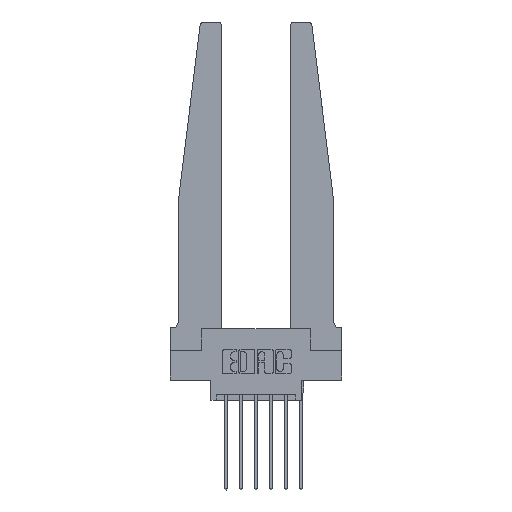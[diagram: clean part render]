
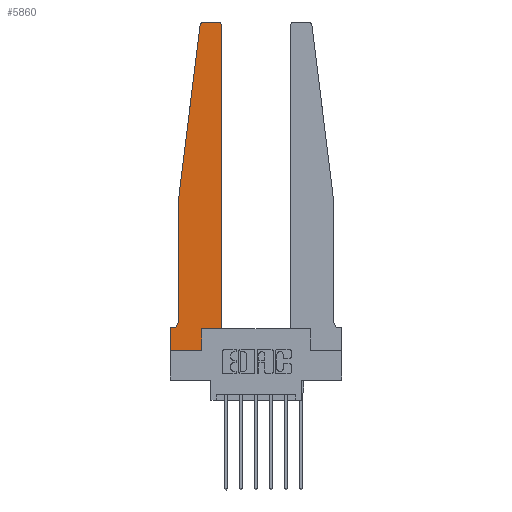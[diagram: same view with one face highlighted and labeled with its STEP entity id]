
A CAD part, top view. The second image highlights one B-rep face of the part: STEP entity #5860.
In plain terms, the highlighted planar face has unit normal (0, 0, 1).
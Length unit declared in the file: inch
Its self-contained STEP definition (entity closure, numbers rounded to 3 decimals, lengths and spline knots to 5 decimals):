
#314 = CIRCLE ( 'NONE', #8016, 0.03 ) ;
#333 = CARTESIAN_POINT ( 'NONE',  ( 0.24675, 2.72367, 0.37 ) ) ;
#404 = VERTEX_POINT ( 'NONE', #2735 ) ;
#415 = ORIENTED_EDGE ( 'NONE', *, *, #5354, .T. ) ;
#635 = DIRECTION ( 'NONE',  ( 0., 0., 1. ) ) ;
#674 = EDGE_CURVE ( 'NONE', #12169, #11411, #849, .T. ) ;
#849 = CIRCLE ( 'NONE', #8551, 0.03 ) ;
#889 = CARTESIAN_POINT ( 'NONE',  ( 0., 0.1875, 0.37 ) ) ;
#920 = VECTOR ( 'NONE', #7276, 39.37008 ) ;
#926 = CARTESIAN_POINT ( 'NONE',  ( 0.015, 0.2375, 0.37 ) ) ;
#1264 = EDGE_CURVE ( 'NONE', #7912, #12169, #11225, .T. ) ;
#1346 = ORIENTED_EDGE ( 'NONE', *, *, #674, .T. ) ;
#1358 = AXIS2_PLACEMENT_3D ( 'NONE', #926, #13428, #7123 ) ;
#1378 = CARTESIAN_POINT ( 'NONE',  ( 0.2605, 0.18, 0.37 ) ) ;
#1619 = LINE ( 'NONE', #10051, #3954 ) ;
#1695 = DIRECTION ( 'NONE',  ( -0.122, -0.992, 0. ) ) ;
#1724 = LINE ( 'NONE', #10158, #8013 ) ;
#1923 = DIRECTION ( 'NONE',  ( 0., 0., 1. ) ) ;
#2057 = FACE_OUTER_BOUND ( 'NONE', #11033, .T. ) ;
#2199 = VERTEX_POINT ( 'NONE', #4110 ) ;
#2253 = DIRECTION ( 'NONE',  ( 1., 0., 0. ) ) ;
#2413 = DIRECTION ( 'NONE',  ( 0., 1., 0. ) ) ;
#2567 = DIRECTION ( 'NONE',  ( 0., -1., 0. ) ) ;
#2568 = CARTESIAN_POINT ( 'NONE',  ( 0.2605, 0., 0.37 ) ) ;
#2637 = LINE ( 'NONE', #3870, #7713 ) ;
#2700 = ORIENTED_EDGE ( 'NONE', *, *, #9136, .T. ) ;
#2715 = LINE ( 'NONE', #3741, #9560 ) ;
#2735 = CARTESIAN_POINT ( 'NONE',  ( 0., 0., 0.37 ) ) ;
#2786 = ORIENTED_EDGE ( 'NONE', *, *, #4569, .T. ) ;
#2891 = CARTESIAN_POINT ( 'NONE',  ( 0.2605, 0.18, 0.37 ) ) ;
#3127 = CARTESIAN_POINT ( 'NONE',  ( 0.27653, 2.75, 0.37 ) ) ;
#3148 = PLANE ( 'NONE',  #8619 ) ;
#3382 = ORIENTED_EDGE ( 'NONE', *, *, #9027, .T. ) ;
#3513 = VECTOR ( 'NONE', #13382, 39.37008 ) ;
#3741 = CARTESIAN_POINT ( 'NONE',  ( 0.425, 0.18, 0.37 ) ) ;
#3796 = CARTESIAN_POINT ( 'NONE',  ( 0.27653, 2.72, 0.37 ) ) ;
#3854 = ORIENTED_EDGE ( 'NONE', *, *, #1264, .T. ) ;
#3870 = CARTESIAN_POINT ( 'NONE',  ( 0.065, 1.25, 0.37 ) ) ;
#3954 = VECTOR ( 'NONE', #2567, 39.37008 ) ;
#4041 = CARTESIAN_POINT ( 'NONE',  ( 0., 0.1875, 0.37 ) ) ;
#4102 = DIRECTION ( 'NONE',  ( 0., 0., 1. ) ) ;
#4110 = CARTESIAN_POINT ( 'NONE',  ( 0.425, 0.18, 0.37 ) ) ;
#4569 = EDGE_CURVE ( 'NONE', #5916, #404, #1619, .T. ) ;
#4619 = EDGE_CURVE ( 'NONE', #11189, #12690, #2637, .T. ) ;
#4818 = LINE ( 'NONE', #11382, #6033 ) ;
#4831 = DIRECTION ( 'NONE',  ( 1., 0., 0. ) ) ;
#5354 = EDGE_CURVE ( 'NONE', #12690, #12303, #10393, .T. ) ;
#5358 = CARTESIAN_POINT ( 'NONE',  ( 0.395, 2.72, 0.37 ) ) ;
#5711 = EDGE_CURVE ( 'NONE', #12443, #11377, #12017, .T. ) ;
#5774 = ORIENTED_EDGE ( 'NONE', *, *, #12333, .T. ) ;
#5860 = ADVANCED_FACE ( 'NONE', ( #2057 ), #3148, .T. ) ;
#5876 = DIRECTION ( 'NONE',  ( 0., -1., 0. ) ) ;
#5877 = DIRECTION ( 'NONE',  ( 0., 1., 0. ) ) ;
#5916 = VERTEX_POINT ( 'NONE', #4041 ) ;
#5963 = CARTESIAN_POINT ( 'NONE',  ( 0.065, 1.25, 0.37 ) ) ;
#6033 = VECTOR ( 'NONE', #13664, 39.37008 ) ;
#6263 = EDGE_CURVE ( 'NONE', #11377, #2199, #12470, .T. ) ;
#6335 = VERTEX_POINT ( 'NONE', #9221 ) ;
#7123 = DIRECTION ( 'NONE',  ( -1., 0., 0. ) ) ;
#7276 = DIRECTION ( 'NONE',  ( 1., 0., 0. ) ) ;
#7650 = EDGE_CURVE ( 'NONE', #11411, #11189, #9139, .T. ) ;
#7713 = VECTOR ( 'NONE', #5876, 39.37008 ) ;
#7912 = VERTEX_POINT ( 'NONE', #9551 ) ;
#7988 = DIRECTION ( 'NONE',  ( -1., 0., 0. ) ) ;
#8013 = VECTOR ( 'NONE', #7988, 39.37008 ) ;
#8016 = AXIS2_PLACEMENT_3D ( 'NONE', #5358, #4102, #2253 ) ;
#8194 = DIRECTION ( 'NONE',  ( 1., 0., 0. ) ) ;
#8215 = CARTESIAN_POINT ( 'NONE',  ( 0.065, 1.25, 0.37 ) ) ;
#8289 = ORIENTED_EDGE ( 'NONE', *, *, #4619, .T. ) ;
#8392 = ORIENTED_EDGE ( 'NONE', *, *, #12643, .T. ) ;
#8551 = AXIS2_PLACEMENT_3D ( 'NONE', #3796, #635, #4831 ) ;
#8619 = AXIS2_PLACEMENT_3D ( 'NONE', #889, #1923, #8194 ) ;
#9027 = EDGE_CURVE ( 'NONE', #12303, #5916, #1724, .T. ) ;
#9136 = EDGE_CURVE ( 'NONE', #404, #12443, #4818, .T. ) ;
#9139 = LINE ( 'NONE', #5963, #13528 ) ;
#9221 = CARTESIAN_POINT ( 'NONE',  ( 0.425, 2.72, 0.37 ) ) ;
#9336 = ORIENTED_EDGE ( 'NONE', *, *, #5711, .T. ) ;
#9551 = CARTESIAN_POINT ( 'NONE',  ( 0.395, 2.75, 0.37 ) ) ;
#9560 = VECTOR ( 'NONE', #5877, 39.37008 ) ;
#9656 = CARTESIAN_POINT ( 'NONE',  ( 0.065, 0.2375, 0.37 ) ) ;
#10051 = CARTESIAN_POINT ( 'NONE',  ( 0., 0., 0.37 ) ) ;
#10158 = CARTESIAN_POINT ( 'NONE',  ( 0.065, 0.1875, 0.37 ) ) ;
#10280 = ORIENTED_EDGE ( 'NONE', *, *, #6263, .T. ) ;
#10393 = CIRCLE ( 'NONE', #1358, 0.05 ) ;
#10534 = ORIENTED_EDGE ( 'NONE', *, *, #7650, .T. ) ;
#10719 = CARTESIAN_POINT ( 'NONE',  ( 0.015, 0.1875, 0.37 ) ) ;
#11033 = EDGE_LOOP ( 'NONE', ( #3854, #1346, #10534, #8289, #415, #3382, #2786, #2700, #9336, #10280, #5774, #8392 ) ) ;
#11158 = CARTESIAN_POINT ( 'NONE',  ( 0.25, 2.75, 0.37 ) ) ;
#11189 = VERTEX_POINT ( 'NONE', #8215 ) ;
#11225 = LINE ( 'NONE', #11158, #3513 ) ;
#11377 = VERTEX_POINT ( 'NONE', #1378 ) ;
#11382 = CARTESIAN_POINT ( 'NONE',  ( 0., 0., 0.37 ) ) ;
#11411 = VERTEX_POINT ( 'NONE', #333 ) ;
#11923 = VECTOR ( 'NONE', #2413, 39.37008 ) ;
#12017 = LINE ( 'NONE', #2891, #11923 ) ;
#12169 = VERTEX_POINT ( 'NONE', #3127 ) ;
#12303 = VERTEX_POINT ( 'NONE', #10719 ) ;
#12333 = EDGE_CURVE ( 'NONE', #2199, #6335, #2715, .T. ) ;
#12443 = VERTEX_POINT ( 'NONE', #2568 ) ;
#12470 = LINE ( 'NONE', #13588, #920 ) ;
#12643 = EDGE_CURVE ( 'NONE', #6335, #7912, #314, .T. ) ;
#12690 = VERTEX_POINT ( 'NONE', #9656 ) ;
#13382 = DIRECTION ( 'NONE',  ( -1., 0., 0. ) ) ;
#13428 = DIRECTION ( 'NONE',  ( 0., 0., -1. ) ) ;
#13528 = VECTOR ( 'NONE', #1695, 39.37008 ) ;
#13588 = CARTESIAN_POINT ( 'NONE',  ( 0.425, 0.18, 0.37 ) ) ;
#13664 = DIRECTION ( 'NONE',  ( 1., 0., 0. ) ) ;
